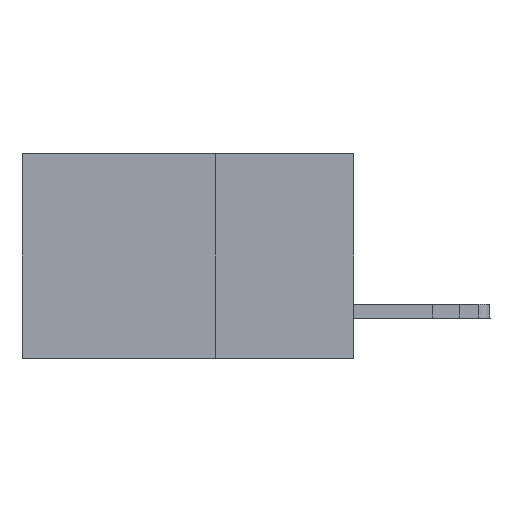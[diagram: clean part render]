
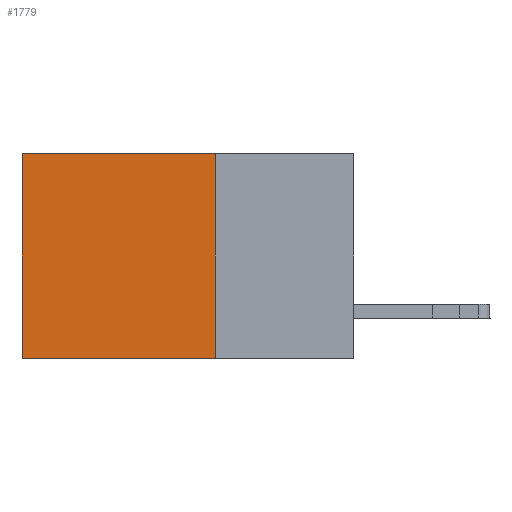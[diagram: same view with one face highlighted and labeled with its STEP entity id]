
A CAD part, left-side view. The second image highlights one B-rep face of the part: STEP entity #1779.
In plain terms, the highlighted planar face has unit normal (-1, 0, 0).
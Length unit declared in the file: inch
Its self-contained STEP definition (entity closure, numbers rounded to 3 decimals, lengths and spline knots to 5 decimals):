
#97 = CARTESIAN_POINT ( 'NONE',  ( 0.2875, 0.6, 0. ) ) ;
#446 = LINE ( 'NONE', #16666, #14859 ) ;
#1130 = ORIENTED_EDGE ( 'NONE', *, *, #16376, .T. ) ;
#1779 = ADVANCED_FACE ( 'NONE', ( #8445 ), #12152, .F. ) ;
#1804 = CARTESIAN_POINT ( 'NONE',  ( 0.2875, 0.6, -0.37 ) ) ;
#2292 = CARTESIAN_POINT ( 'NONE',  ( 0.2875, 0.25, 0. ) ) ;
#3241 = CARTESIAN_POINT ( 'NONE',  ( 0.2875, 0.25, 0. ) ) ;
#4362 = VERTEX_POINT ( 'NONE', #10294 ) ;
#5831 = LINE ( 'NONE', #9543, #12557 ) ;
#6520 = DIRECTION ( 'NONE',  ( 0., 0., -1. ) ) ;
#6741 = LINE ( 'NONE', #18908, #15001 ) ;
#6833 = EDGE_LOOP ( 'NONE', ( #1130, #23227, #17431, #16422 ) ) ;
#8445 = FACE_OUTER_BOUND ( 'NONE', #6833, .T. ) ;
#8550 = CARTESIAN_POINT ( 'NONE',  ( 0.2875, 0.6, 0. ) ) ;
#9543 = CARTESIAN_POINT ( 'NONE',  ( 0.2875, 0.25, 0. ) ) ;
#10294 = CARTESIAN_POINT ( 'NONE',  ( 0.2875, 0.25, -0.37 ) ) ;
#11352 = VERTEX_POINT ( 'NONE', #8550 ) ;
#12152 = PLANE ( 'NONE',  #21145 ) ;
#12557 = VECTOR ( 'NONE', #18934, 39.37008 ) ;
#13357 = DIRECTION ( 'NONE',  ( 0., 1., 0. ) ) ;
#14859 = VECTOR ( 'NONE', #13357, 39.37008 ) ;
#15001 = VECTOR ( 'NONE', #23488, 39.37008 ) ;
#15054 = DIRECTION ( 'NONE',  ( 1., 0., 0. ) ) ;
#15185 = VERTEX_POINT ( 'NONE', #3241 ) ;
#15954 = DIRECTION ( 'NONE',  ( 0., 0., -1. ) ) ;
#16043 = VERTEX_POINT ( 'NONE', #1804 ) ;
#16376 = EDGE_CURVE ( 'NONE', #11352, #16043, #16431, .T. ) ;
#16422 = ORIENTED_EDGE ( 'NONE', *, *, #20816, .T. ) ;
#16431 = LINE ( 'NONE', #97, #16486 ) ;
#16486 = VECTOR ( 'NONE', #15954, 39.37008 ) ;
#16666 = CARTESIAN_POINT ( 'NONE',  ( 0.2875, 0.25, 0. ) ) ;
#17431 = ORIENTED_EDGE ( 'NONE', *, *, #20413, .F. ) ;
#18512 = EDGE_CURVE ( 'NONE', #4362, #16043, #6741, .T. ) ;
#18908 = CARTESIAN_POINT ( 'NONE',  ( 0.2875, 0.25, -0.37 ) ) ;
#18934 = DIRECTION ( 'NONE',  ( 0., 0., -1. ) ) ;
#20413 = EDGE_CURVE ( 'NONE', #15185, #4362, #5831, .T. ) ;
#20816 = EDGE_CURVE ( 'NONE', #15185, #11352, #446, .T. ) ;
#21145 = AXIS2_PLACEMENT_3D ( 'NONE', #2292, #15054, #6520 ) ;
#23227 = ORIENTED_EDGE ( 'NONE', *, *, #18512, .F. ) ;
#23488 = DIRECTION ( 'NONE',  ( 0., 1., 0. ) ) ;
